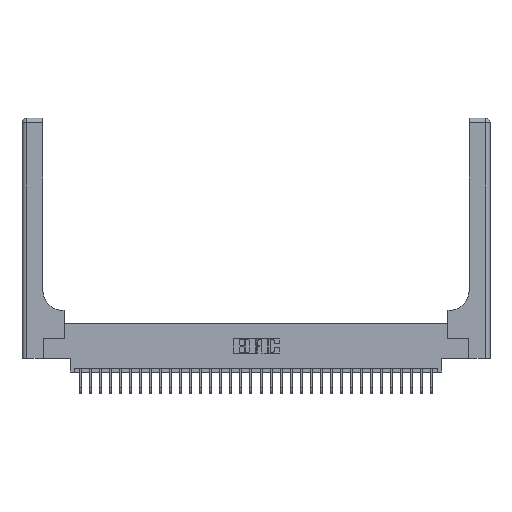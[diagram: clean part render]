
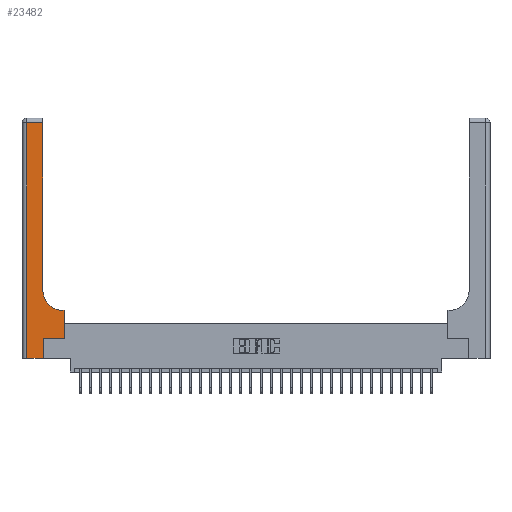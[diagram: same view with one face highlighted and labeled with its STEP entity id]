
A CAD part, top view. The second image highlights one B-rep face of the part: STEP entity #23482.
In plain terms, the highlighted planar face has unit normal (0, 0, 1).
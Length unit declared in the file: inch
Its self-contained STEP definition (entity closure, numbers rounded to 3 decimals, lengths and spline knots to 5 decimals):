
#100 = DIRECTION ( 'NONE',  ( -1., 0., 0. ) ) ;
#378 = CARTESIAN_POINT ( 'NONE',  ( 0., 3., 0.37 ) ) ;
#1148 = LINE ( 'NONE', #10678, #4543 ) ;
#1820 = VERTEX_POINT ( 'NONE', #24956 ) ;
#1857 = VECTOR ( 'NONE', #5746, 39.37008 ) ;
#1878 = EDGE_LOOP ( 'NONE', ( #12856, #14858, #24946, #14561, #8164, #23662, #9517, #25869, #26822 ) ) ;
#2350 = DIRECTION ( 'NONE',  ( 1., 0., 0. ) ) ;
#2539 = VERTEX_POINT ( 'NONE', #23894 ) ;
#2776 = CARTESIAN_POINT ( 'NONE',  ( 0.51, 0.85, 0.37 ) ) ;
#3240 = EDGE_CURVE ( 'NONE', #4029, #6880, #14579, .T. ) ;
#3728 = VERTEX_POINT ( 'NONE', #24009 ) ;
#4029 = VERTEX_POINT ( 'NONE', #19095 ) ;
#4408 = VECTOR ( 'NONE', #100, 39.37008 ) ;
#4543 = VECTOR ( 'NONE', #21003, 39.37008 ) ;
#5746 = DIRECTION ( 'NONE',  ( 0., 1., 0. ) ) ;
#6272 = DIRECTION ( 'NONE',  ( 1., 0., 0. ) ) ;
#6495 = CARTESIAN_POINT ( 'NONE',  ( 0.06, 2.94, 0.37 ) ) ;
#6765 = EDGE_CURVE ( 'NONE', #26069, #18154, #10607, .T. ) ;
#6880 = VERTEX_POINT ( 'NONE', #25085 ) ;
#7554 = DIRECTION ( 'NONE',  ( 0., 1., 0. ) ) ;
#8042 = VERTEX_POINT ( 'NONE', #15137 ) ;
#8164 = ORIENTED_EDGE ( 'NONE', *, *, #17196, .T. ) ;
#9111 = AXIS2_PLACEMENT_3D ( 'NONE', #378, #9369, #11953 ) ;
#9369 = DIRECTION ( 'NONE',  ( 0., 0., -1. ) ) ;
#9517 = ORIENTED_EDGE ( 'NONE', *, *, #3240, .T. ) ;
#10312 = EDGE_CURVE ( 'NONE', #18154, #8042, #1148, .T. ) ;
#10607 = LINE ( 'NONE', #22197, #27330 ) ;
#10678 = CARTESIAN_POINT ( 'NONE',  ( 0., 0., 0.37 ) ) ;
#10679 = VECTOR ( 'NONE', #6272, 39.37008 ) ;
#10839 = DIRECTION ( 'NONE',  ( 0., 1., 0. ) ) ;
#11953 = DIRECTION ( 'NONE',  ( -1., 0., 0. ) ) ;
#11966 = CARTESIAN_POINT ( 'NONE',  ( 0.06, 0., 0.37 ) ) ;
#12136 = EDGE_CURVE ( 'NONE', #2539, #3728, #26545, .T. ) ;
#12740 = VERTEX_POINT ( 'NONE', #28271 ) ;
#12856 = ORIENTED_EDGE ( 'NONE', *, *, #27366, .T. ) ;
#12881 = CARTESIAN_POINT ( 'NONE',  ( 0.26, 3., 0.37 ) ) ;
#13423 = VECTOR ( 'NONE', #27930, 39.37008 ) ;
#13883 = FACE_OUTER_BOUND ( 'NONE', #1878, .T. ) ;
#14561 = ORIENTED_EDGE ( 'NONE', *, *, #10312, .T. ) ;
#14579 = LINE ( 'NONE', #23525, #18646 ) ;
#14858 = ORIENTED_EDGE ( 'NONE', *, *, #23483, .T. ) ;
#15137 = CARTESIAN_POINT ( 'NONE',  ( 0.265, 0., 0.37 ) ) ;
#15187 = LINE ( 'NONE', #24125, #13423 ) ;
#16890 = LINE ( 'NONE', #17166, #1857 ) ;
#17166 = CARTESIAN_POINT ( 'NONE',  ( 0.265, 0., 0.37 ) ) ;
#17196 = EDGE_CURVE ( 'NONE', #8042, #12740, #16890, .T. ) ;
#17365 = DIRECTION ( 'NONE',  ( 0., -1., 0. ) ) ;
#18154 = VERTEX_POINT ( 'NONE', #11966 ) ;
#18434 = CARTESIAN_POINT ( 'NONE',  ( 0., 2.94, 0.37 ) ) ;
#18646 = VECTOR ( 'NONE', #7554, 39.37008 ) ;
#19095 = CARTESIAN_POINT ( 'NONE',  ( 0.528, 0.25, 0.37 ) ) ;
#21003 = DIRECTION ( 'NONE',  ( 1., 0., 0. ) ) ;
#21995 = LINE ( 'NONE', #12881, #26055 ) ;
#22197 = CARTESIAN_POINT ( 'NONE',  ( 0.06, 3., 0.37 ) ) ;
#22848 = LINE ( 'NONE', #18434, #4408 ) ;
#23482 = ADVANCED_FACE ( 'NONE', ( #13883 ), #25026, .F. ) ;
#23483 = EDGE_CURVE ( 'NONE', #1820, #26069, #22848, .T. ) ;
#23525 = CARTESIAN_POINT ( 'NONE',  ( 0.528, 0.25, 0.37 ) ) ;
#23662 = ORIENTED_EDGE ( 'NONE', *, *, #28739, .T. ) ;
#23894 = CARTESIAN_POINT ( 'NONE',  ( 0.51, 0.6, 0.37 ) ) ;
#24009 = CARTESIAN_POINT ( 'NONE',  ( 0.26, 0.85, 0.37 ) ) ;
#24125 = CARTESIAN_POINT ( 'NONE',  ( 0.26, 0.6, 0.37 ) ) ;
#24946 = ORIENTED_EDGE ( 'NONE', *, *, #6765, .T. ) ;
#24956 = CARTESIAN_POINT ( 'NONE',  ( 0.26, 2.94, 0.37 ) ) ;
#25026 = PLANE ( 'NONE',  #9111 ) ;
#25085 = CARTESIAN_POINT ( 'NONE',  ( 0.528, 0.6, 0.37 ) ) ;
#25869 = ORIENTED_EDGE ( 'NONE', *, *, #27537, .T. ) ;
#26055 = VECTOR ( 'NONE', #10839, 39.37008 ) ;
#26069 = VERTEX_POINT ( 'NONE', #6495 ) ;
#26349 = CARTESIAN_POINT ( 'NONE',  ( 0.265, 0.25, 0.37 ) ) ;
#26545 = CIRCLE ( 'NONE', #27958, 0.25 ) ;
#26822 = ORIENTED_EDGE ( 'NONE', *, *, #12136, .T. ) ;
#26824 = DIRECTION ( 'NONE',  ( 0., 0., -1. ) ) ;
#27330 = VECTOR ( 'NONE', #17365, 39.37008 ) ;
#27366 = EDGE_CURVE ( 'NONE', #3728, #1820, #21995, .T. ) ;
#27537 = EDGE_CURVE ( 'NONE', #6880, #2539, #15187, .T. ) ;
#27930 = DIRECTION ( 'NONE',  ( -1., 0., 0. ) ) ;
#27958 = AXIS2_PLACEMENT_3D ( 'NONE', #2776, #26824, #2350 ) ;
#28271 = CARTESIAN_POINT ( 'NONE',  ( 0.265, 0.25, 0.37 ) ) ;
#28554 = LINE ( 'NONE', #26349, #10679 ) ;
#28739 = EDGE_CURVE ( 'NONE', #12740, #4029, #28554, .T. ) ;
